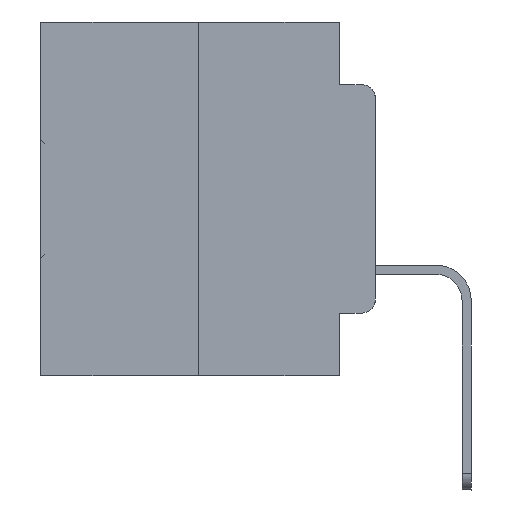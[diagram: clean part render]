
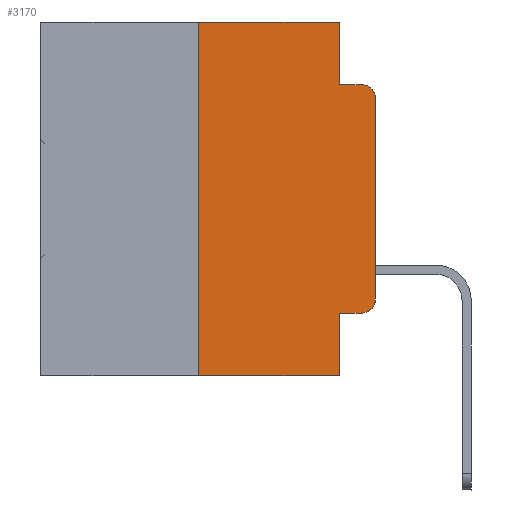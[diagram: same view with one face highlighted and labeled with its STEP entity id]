
A CAD part, left-side view. The second image highlights one B-rep face of the part: STEP entity #3170.
In plain terms, the highlighted planar face has unit normal (-1, 0, 0).
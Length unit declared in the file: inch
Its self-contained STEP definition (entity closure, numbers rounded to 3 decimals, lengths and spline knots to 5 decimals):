
#876 = ORIENTED_EDGE ( 'NONE', *, *, #12079, .F. ) ;
#1757 = DIRECTION ( 'NONE',  ( 0., -1., 0. ) ) ;
#2054 = ORIENTED_EDGE ( 'NONE', *, *, #13167, .F. ) ;
#2424 = CARTESIAN_POINT ( 'NONE',  ( 0., 0.051, -0.0885 ) ) ;
#2718 = LINE ( 'NONE', #16293, #11513 ) ;
#2839 = DIRECTION ( 'NONE',  ( -1., 0., 0. ) ) ;
#3170 = ADVANCED_FACE ( 'NONE', ( #6296 ), #13576, .F. ) ;
#3755 = CARTESIAN_POINT ( 'NONE',  ( 0., 0.02, -0.0885 ) ) ;
#3814 = CARTESIAN_POINT ( 'NONE',  ( 0., 0., -0.3915 ) ) ;
#4734 = ORIENTED_EDGE ( 'NONE', *, *, #5300, .T. ) ;
#4774 = ORIENTED_EDGE ( 'NONE', *, *, #13397, .F. ) ;
#4831 = DIRECTION ( 'NONE',  ( 0., -1., 0. ) ) ;
#5114 = CARTESIAN_POINT ( 'NONE',  ( 0., 0.25, -0.5 ) ) ;
#5300 = EDGE_CURVE ( 'NONE', #22620, #24689, #6180, .T. ) ;
#6180 = LINE ( 'NONE', #24588, #28786 ) ;
#6296 = FACE_OUTER_BOUND ( 'NONE', #31271, .T. ) ;
#6497 = ORIENTED_EDGE ( 'NONE', *, *, #8043, .T. ) ;
#6940 = CARTESIAN_POINT ( 'NONE',  ( 0., 0.473, -0.5 ) ) ;
#7727 = CARTESIAN_POINT ( 'NONE',  ( 0., 0.02, -0.3915 ) ) ;
#7748 = CIRCLE ( 'NONE', #22376, 0.02 ) ;
#8043 = EDGE_CURVE ( 'NONE', #22060, #22675, #16820, .T. ) ;
#8302 = DIRECTION ( 'NONE',  ( -1., 0., 0. ) ) ;
#8618 = CARTESIAN_POINT ( 'NONE',  ( 0., 0.473, 0. ) ) ;
#8967 = EDGE_CURVE ( 'NONE', #24689, #14878, #24375, .T. ) ;
#9676 = AXIS2_PLACEMENT_3D ( 'NONE', #22795, #8302, #10571 ) ;
#10571 = DIRECTION ( 'NONE',  ( 0., 0., -1. ) ) ;
#11102 = DIRECTION ( 'NONE',  ( 0., 0., -1. ) ) ;
#11167 = DIRECTION ( 'NONE',  ( 0., 0., -1. ) ) ;
#11513 = VECTOR ( 'NONE', #1757, 39.37008 ) ;
#12079 = EDGE_CURVE ( 'NONE', #19635, #21156, #25747, .T. ) ;
#13167 = EDGE_CURVE ( 'NONE', #20515, #19635, #2718, .T. ) ;
#13190 = CARTESIAN_POINT ( 'NONE',  ( 0., 0.051, 0. ) ) ;
#13397 = EDGE_CURVE ( 'NONE', #21156, #14878, #15515, .T. ) ;
#13576 = PLANE ( 'NONE',  #24133 ) ;
#14149 = CARTESIAN_POINT ( 'NONE',  ( 0., 0.051, -0.5 ) ) ;
#14757 = CARTESIAN_POINT ( 'NONE',  ( 0., 0.051, -0.0885 ) ) ;
#14878 = VERTEX_POINT ( 'NONE', #3755 ) ;
#14996 = ORIENTED_EDGE ( 'NONE', *, *, #21294, .T. ) ;
#15515 = LINE ( 'NONE', #14757, #15909 ) ;
#15909 = VECTOR ( 'NONE', #4831, 39.37008 ) ;
#16293 = CARTESIAN_POINT ( 'NONE',  ( 0., 0.473, 0. ) ) ;
#16780 = ORIENTED_EDGE ( 'NONE', *, *, #28911, .F. ) ;
#16820 = LINE ( 'NONE', #21243, #21788 ) ;
#16938 = VERTEX_POINT ( 'NONE', #14149 ) ;
#17262 = LINE ( 'NONE', #6940, #17686 ) ;
#17327 = DIRECTION ( 'NONE',  ( 0., -1., 0. ) ) ;
#17686 = VECTOR ( 'NONE', #17327, 39.37008 ) ;
#17948 = DIRECTION ( 'NONE',  ( 0., 0., -1. ) ) ;
#18347 = CARTESIAN_POINT ( 'NONE',  ( 0., 0.25, 0. ) ) ;
#18572 = DIRECTION ( 'NONE',  ( 0., 0., 1. ) ) ;
#18683 = DIRECTION ( 'NONE',  ( 0., -1., 0. ) ) ;
#18795 = VERTEX_POINT ( 'NONE', #5114 ) ;
#19635 = VERTEX_POINT ( 'NONE', #13190 ) ;
#19737 = ORIENTED_EDGE ( 'NONE', *, *, #22221, .T. ) ;
#20283 = LINE ( 'NONE', #18347, #27916 ) ;
#20515 = VERTEX_POINT ( 'NONE', #28977 ) ;
#21093 = CARTESIAN_POINT ( 'NONE',  ( 0., 0.051, -0.4115 ) ) ;
#21156 = VERTEX_POINT ( 'NONE', #2424 ) ;
#21243 = CARTESIAN_POINT ( 'NONE',  ( 0., 0.051, -0.4115 ) ) ;
#21294 = EDGE_CURVE ( 'NONE', #22675, #22620, #7748, .T. ) ;
#21677 = ORIENTED_EDGE ( 'NONE', *, *, #23289, .F. ) ;
#21788 = VECTOR ( 'NONE', #18683, 39.37008 ) ;
#22016 = LINE ( 'NONE', #30296, #30067 ) ;
#22060 = VERTEX_POINT ( 'NONE', #21093 ) ;
#22221 = EDGE_CURVE ( 'NONE', #18795, #16938, #17262, .T. ) ;
#22376 = AXIS2_PLACEMENT_3D ( 'NONE', #7727, #2839, #24977 ) ;
#22620 = VERTEX_POINT ( 'NONE', #3814 ) ;
#22675 = VERTEX_POINT ( 'NONE', #26079 ) ;
#22795 = CARTESIAN_POINT ( 'NONE',  ( 0., 0.02, -0.1085 ) ) ;
#23289 = EDGE_CURVE ( 'NONE', #18795, #20515, #20283, .T. ) ;
#24133 = AXIS2_PLACEMENT_3D ( 'NONE', #8618, #30572, #11102 ) ;
#24375 = CIRCLE ( 'NONE', #9676, 0.02 ) ;
#24588 = CARTESIAN_POINT ( 'NONE',  ( 0., 0., 0. ) ) ;
#24689 = VERTEX_POINT ( 'NONE', #28166 ) ;
#24977 = DIRECTION ( 'NONE',  ( 0., 0., -1. ) ) ;
#25747 = LINE ( 'NONE', #28399, #29923 ) ;
#26079 = CARTESIAN_POINT ( 'NONE',  ( 0., 0.02, -0.4115 ) ) ;
#26882 = ORIENTED_EDGE ( 'NONE', *, *, #8967, .T. ) ;
#27163 = DIRECTION ( 'NONE',  ( 0., 0., 1. ) ) ;
#27916 = VECTOR ( 'NONE', #18572, 39.37008 ) ;
#28166 = CARTESIAN_POINT ( 'NONE',  ( 0., 0., -0.1085 ) ) ;
#28399 = CARTESIAN_POINT ( 'NONE',  ( 0., 0.051, 0. ) ) ;
#28786 = VECTOR ( 'NONE', #27163, 39.37008 ) ;
#28911 = EDGE_CURVE ( 'NONE', #22060, #16938, #22016, .T. ) ;
#28977 = CARTESIAN_POINT ( 'NONE',  ( 0., 0.25, 0. ) ) ;
#29923 = VECTOR ( 'NONE', #11167, 39.37008 ) ;
#30067 = VECTOR ( 'NONE', #17948, 39.37008 ) ;
#30296 = CARTESIAN_POINT ( 'NONE',  ( 0., 0.051, 0. ) ) ;
#30572 = DIRECTION ( 'NONE',  ( 1., 0., 0. ) ) ;
#31271 = EDGE_LOOP ( 'NONE', ( #4734, #26882, #4774, #876, #2054, #21677, #19737, #16780, #6497, #14996 ) ) ;
